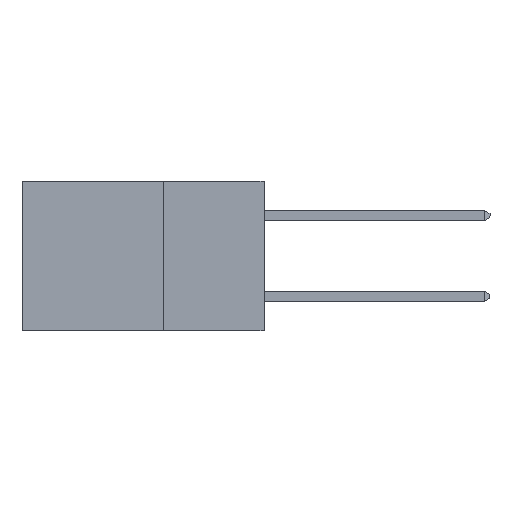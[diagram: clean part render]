
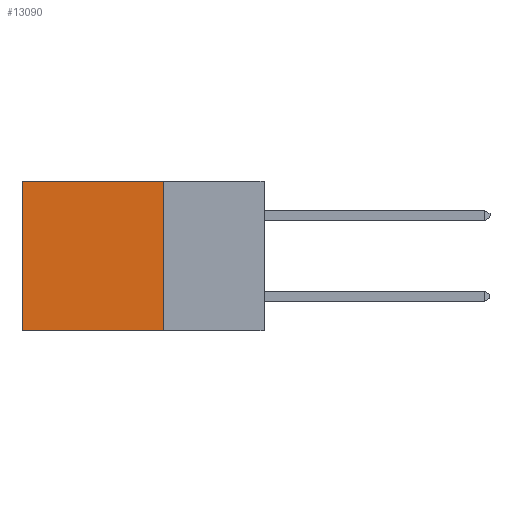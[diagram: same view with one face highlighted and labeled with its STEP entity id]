
A CAD part, left-side view. The second image highlights one B-rep face of the part: STEP entity #13090.
In plain terms, the highlighted planar face has unit normal (-1, 0, 0).
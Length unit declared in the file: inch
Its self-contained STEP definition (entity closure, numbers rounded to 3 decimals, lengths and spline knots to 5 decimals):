
#134 = ORIENTED_EDGE ( 'NONE', *, *, #27883, .T. ) ;
#1101 = VERTEX_POINT ( 'NONE', #24052 ) ;
#1488 = DIRECTION ( 'NONE',  ( 0., 0., -1. ) ) ;
#1687 = ORIENTED_EDGE ( 'NONE', *, *, #22151, .T. ) ;
#3221 = FACE_OUTER_BOUND ( 'NONE', #4849, .T. ) ;
#4487 = CARTESIAN_POINT ( 'NONE',  ( 0.298, 0.25, 0. ) ) ;
#4849 = EDGE_LOOP ( 'NONE', ( #134, #7391, #17379, #1687 ) ) ;
#5305 = LINE ( 'NONE', #20540, #17543 ) ;
#5722 = VERTEX_POINT ( 'NONE', #4487 ) ;
#6250 = CARTESIAN_POINT ( 'NONE',  ( 0.298, 0.6, 0. ) ) ;
#6638 = LINE ( 'NONE', #20905, #21202 ) ;
#7391 = ORIENTED_EDGE ( 'NONE', *, *, #12634, .F. ) ;
#7459 = AXIS2_PLACEMENT_3D ( 'NONE', #21028, #14569, #1488 ) ;
#8734 = DIRECTION ( 'NONE',  ( 0., 1., 0. ) ) ;
#9086 = VECTOR ( 'NONE', #8734, 39.37008 ) ;
#9653 = DIRECTION ( 'NONE',  ( 0., 0., -1. ) ) ;
#10014 = DIRECTION ( 'NONE',  ( 0., 0., -1. ) ) ;
#10222 = PLANE ( 'NONE',  #7459 ) ;
#12052 = VECTOR ( 'NONE', #23204, 39.37008 ) ;
#12634 = EDGE_CURVE ( 'NONE', #26021, #1101, #26976, .T. ) ;
#13090 = ADVANCED_FACE ( 'NONE', ( #3221 ), #10222, .F. ) ;
#14569 = DIRECTION ( 'NONE',  ( 1., 0., 0. ) ) ;
#14596 = VERTEX_POINT ( 'NONE', #6250 ) ;
#16055 = CARTESIAN_POINT ( 'NONE',  ( 0.298, 0.25, -0.37 ) ) ;
#17379 = ORIENTED_EDGE ( 'NONE', *, *, #26044, .F. ) ;
#17543 = VECTOR ( 'NONE', #9653, 39.37008 ) ;
#20540 = CARTESIAN_POINT ( 'NONE',  ( 0.298, 0.25, 0. ) ) ;
#20905 = CARTESIAN_POINT ( 'NONE',  ( 0.298, 0.6, 0. ) ) ;
#21028 = CARTESIAN_POINT ( 'NONE',  ( 0.298, 0.25, 0. ) ) ;
#21202 = VECTOR ( 'NONE', #10014, 39.37008 ) ;
#21701 = CARTESIAN_POINT ( 'NONE',  ( 0.298, 0.25, -0.37 ) ) ;
#22151 = EDGE_CURVE ( 'NONE', #5722, #14596, #23555, .T. ) ;
#23204 = DIRECTION ( 'NONE',  ( 0., 1., 0. ) ) ;
#23555 = LINE ( 'NONE', #27410, #12052 ) ;
#24052 = CARTESIAN_POINT ( 'NONE',  ( 0.298, 0.6, -0.37 ) ) ;
#26021 = VERTEX_POINT ( 'NONE', #16055 ) ;
#26044 = EDGE_CURVE ( 'NONE', #5722, #26021, #5305, .T. ) ;
#26976 = LINE ( 'NONE', #21701, #9086 ) ;
#27410 = CARTESIAN_POINT ( 'NONE',  ( 0.298, 0.25, 0. ) ) ;
#27883 = EDGE_CURVE ( 'NONE', #14596, #1101, #6638, .T. ) ;
